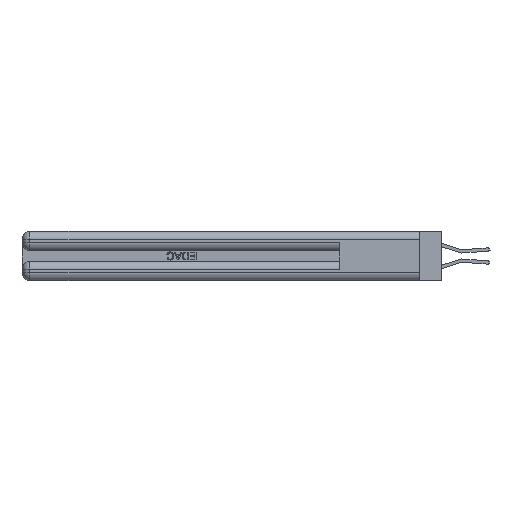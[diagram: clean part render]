
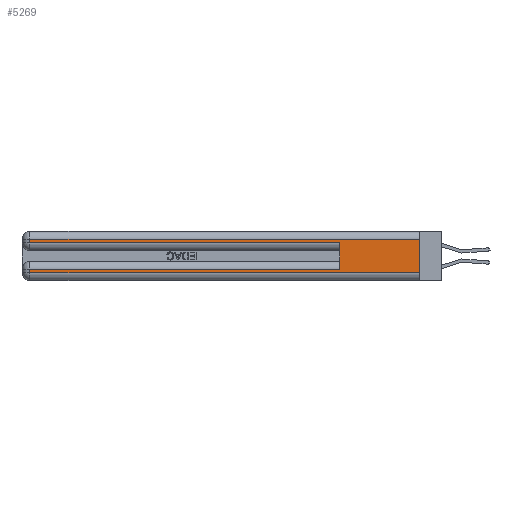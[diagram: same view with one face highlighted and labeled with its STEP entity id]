
A CAD part, left-side view. The second image highlights one B-rep face of the part: STEP entity #5269.
In plain terms, the highlighted planar face has unit normal (-1, 0, 0).
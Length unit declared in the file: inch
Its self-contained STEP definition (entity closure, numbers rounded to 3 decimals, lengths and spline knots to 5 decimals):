
#406 = LINE ( 'NONE', #2243, #27772 ) ;
#571 = VECTOR ( 'NONE', #7997, 39.37008 ) ;
#2243 = CARTESIAN_POINT ( 'NONE',  ( 0., 0., 0.31 ) ) ;
#2495 = DIRECTION ( 'NONE',  ( 1., 0., 0. ) ) ;
#3301 = VECTOR ( 'NONE', #40035, 39.37008 ) ;
#5137 = LINE ( 'NONE', #24735, #41182 ) ;
#5269 = ADVANCED_FACE ( 'NONE', ( #6353 ), #21064, .F. ) ;
#5671 = VECTOR ( 'NONE', #46040, 39.37008 ) ;
#5993 = DIRECTION ( 'NONE',  ( 0., 1., 0. ) ) ;
#6353 = FACE_OUTER_BOUND ( 'NONE', #34500, .T. ) ;
#7014 = CARTESIAN_POINT ( 'NONE',  ( 0., 0., 0.06 ) ) ;
#7271 = CARTESIAN_POINT ( 'NONE',  ( 0., 2.94, 0.31 ) ) ;
#7997 = DIRECTION ( 'NONE',  ( 0., 0., -1. ) ) ;
#10323 = EDGE_CURVE ( 'NONE', #11902, #32583, #38111, .T. ) ;
#10901 = CARTESIAN_POINT ( 'NONE',  ( 0., 0., 0.285 ) ) ;
#11032 = EDGE_CURVE ( 'NONE', #21763, #32583, #47287, .T. ) ;
#11902 = VERTEX_POINT ( 'NONE', #38903 ) ;
#14766 = ORIENTED_EDGE ( 'NONE', *, *, #15071, .T. ) ;
#15071 = EDGE_CURVE ( 'NONE', #21848, #35365, #5137, .T. ) ;
#15545 = DIRECTION ( 'NONE',  ( 0., 0., 1. ) ) ;
#16729 = LINE ( 'NONE', #20245, #5671 ) ;
#17160 = ORIENTED_EDGE ( 'NONE', *, *, #29652, .T. ) ;
#17168 = CARTESIAN_POINT ( 'NONE',  ( 0., 2.94, 0.06 ) ) ;
#19007 = EDGE_CURVE ( 'NONE', #29676, #35365, #42468, .T. ) ;
#20245 = CARTESIAN_POINT ( 'NONE',  ( 0., 2.94, 0.37 ) ) ;
#20472 = EDGE_CURVE ( 'NONE', #21295, #21848, #16729, .T. ) ;
#20473 = LINE ( 'NONE', #37655, #47749 ) ;
#21064 = PLANE ( 'NONE',  #42799 ) ;
#21295 = VERTEX_POINT ( 'NONE', #28287 ) ;
#21763 = VERTEX_POINT ( 'NONE', #46085 ) ;
#21848 = VERTEX_POINT ( 'NONE', #17168 ) ;
#23121 = LINE ( 'NONE', #28824, #3301 ) ;
#24735 = CARTESIAN_POINT ( 'NONE',  ( 0., 0., 0.06 ) ) ;
#26434 = DIRECTION ( 'NONE',  ( 0., 1., 0. ) ) ;
#26546 = CARTESIAN_POINT ( 'NONE',  ( 0., 0., 0.37 ) ) ;
#27575 = VECTOR ( 'NONE', #15545, 39.37008 ) ;
#27772 = VECTOR ( 'NONE', #5993, 39.37008 ) ;
#27775 = ORIENTED_EDGE ( 'NONE', *, *, #19007, .F. ) ;
#28206 = VECTOR ( 'NONE', #47926, 39.37008 ) ;
#28287 = CARTESIAN_POINT ( 'NONE',  ( 0., 2.94, 0.085 ) ) ;
#28431 = CARTESIAN_POINT ( 'NONE',  ( 0., 0., 0.31 ) ) ;
#28446 = DIRECTION ( 'NONE',  ( 0., -1., 0. ) ) ;
#28524 = DIRECTION ( 'NONE',  ( 0., 0., -1. ) ) ;
#28824 = CARTESIAN_POINT ( 'NONE',  ( 0., 2.94, 0.37 ) ) ;
#28878 = ORIENTED_EDGE ( 'NONE', *, *, #36688, .T. ) ;
#29652 = EDGE_CURVE ( 'NONE', #29676, #31693, #406, .T. ) ;
#29676 = VERTEX_POINT ( 'NONE', #28431 ) ;
#31260 = CARTESIAN_POINT ( 'NONE',  ( 0., 0.6, 0.285 ) ) ;
#31693 = VERTEX_POINT ( 'NONE', #7271 ) ;
#32583 = VERTEX_POINT ( 'NONE', #31260 ) ;
#33016 = ORIENTED_EDGE ( 'NONE', *, *, #11032, .F. ) ;
#34500 = EDGE_LOOP ( 'NONE', ( #27775, #17160, #43637, #38424, #33016, #28878, #35662, #14766 ) ) ;
#35365 = VERTEX_POINT ( 'NONE', #7014 ) ;
#35662 = ORIENTED_EDGE ( 'NONE', *, *, #20472, .T. ) ;
#35858 = CARTESIAN_POINT ( 'NONE',  ( 0., 0., 0.37 ) ) ;
#36688 = EDGE_CURVE ( 'NONE', #21763, #21295, #20473, .T. ) ;
#37655 = CARTESIAN_POINT ( 'NONE',  ( 0., 0., 0.085 ) ) ;
#38111 = LINE ( 'NONE', #10901, #28206 ) ;
#38424 = ORIENTED_EDGE ( 'NONE', *, *, #10323, .T. ) ;
#38903 = CARTESIAN_POINT ( 'NONE',  ( 0., 2.94, 0.285 ) ) ;
#40035 = DIRECTION ( 'NONE',  ( 0., 0., -1. ) ) ;
#40336 = EDGE_CURVE ( 'NONE', #31693, #11902, #23121, .T. ) ;
#41182 = VECTOR ( 'NONE', #28446, 39.37008 ) ;
#42468 = LINE ( 'NONE', #26546, #571 ) ;
#42799 = AXIS2_PLACEMENT_3D ( 'NONE', #35858, #2495, #28524 ) ;
#43637 = ORIENTED_EDGE ( 'NONE', *, *, #40336, .T. ) ;
#45291 = CARTESIAN_POINT ( 'NONE',  ( 0., 0.6, 0.145 ) ) ;
#46040 = DIRECTION ( 'NONE',  ( 0., 0., -1. ) ) ;
#46085 = CARTESIAN_POINT ( 'NONE',  ( 0., 0.6, 0.085 ) ) ;
#47287 = LINE ( 'NONE', #45291, #27575 ) ;
#47749 = VECTOR ( 'NONE', #26434, 39.37008 ) ;
#47926 = DIRECTION ( 'NONE',  ( 0., -1., 0. ) ) ;
